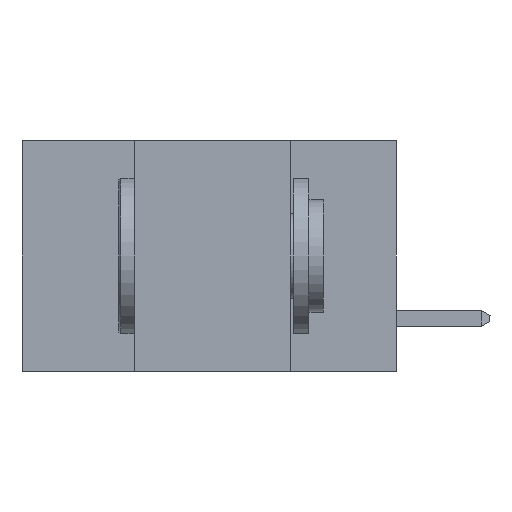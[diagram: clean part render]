
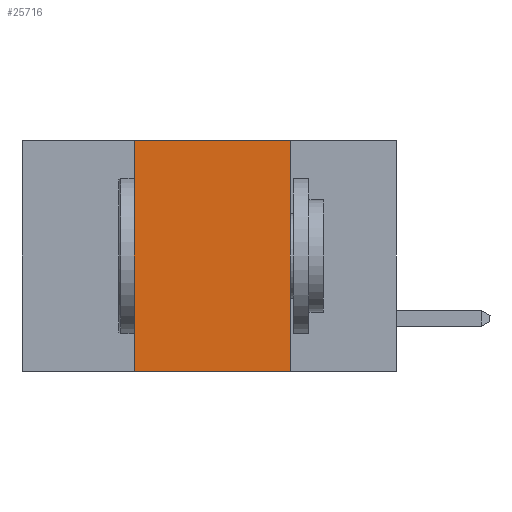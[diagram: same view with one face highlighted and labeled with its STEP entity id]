
A CAD part, left-side view. The second image highlights one B-rep face of the part: STEP entity #25716.
In plain terms, the highlighted planar face has unit normal (-1, 0, 0).
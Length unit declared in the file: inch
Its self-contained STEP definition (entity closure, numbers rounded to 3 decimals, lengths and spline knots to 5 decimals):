
#216 = DIRECTION ( 'NONE',  ( 1., 0., 0. ) ) ;
#978 = EDGE_LOOP ( 'NONE', ( #2393, #16390, #19862, #27914 ) ) ;
#1109 = EDGE_CURVE ( 'NONE', #26123, #24449, #20976, .T. ) ;
#1165 = LINE ( 'NONE', #5066, #31692 ) ;
#2374 = DIRECTION ( 'NONE',  ( 0., 0., -1. ) ) ;
#2393 = ORIENTED_EDGE ( 'NONE', *, *, #22762, .F. ) ;
#3804 = LINE ( 'NONE', #12162, #8048 ) ;
#5066 = CARTESIAN_POINT ( 'NONE',  ( 0., 0.6, 0. ) ) ;
#6222 = AXIS2_PLACEMENT_3D ( 'NONE', #26972, #216, #2374 ) ;
#8048 = VECTOR ( 'NONE', #26833, 39.37008 ) ;
#9158 = FACE_OUTER_BOUND ( 'NONE', #978, .T. ) ;
#9407 = CARTESIAN_POINT ( 'NONE',  ( 0., 0.6, -0.37 ) ) ;
#9566 = EDGE_CURVE ( 'NONE', #30830, #19050, #1165, .T. ) ;
#9730 = PLANE ( 'NONE',  #6222 ) ;
#10147 = VECTOR ( 'NONE', #14366, 39.37008 ) ;
#10358 = CARTESIAN_POINT ( 'NONE',  ( 0., 0.17, 0. ) ) ;
#12120 = DIRECTION ( 'NONE',  ( 0., 0., -1. ) ) ;
#12162 = CARTESIAN_POINT ( 'NONE',  ( 0., 0.42, 0. ) ) ;
#12281 = DIRECTION ( 'NONE',  ( 0., -1., 0. ) ) ;
#14366 = DIRECTION ( 'NONE',  ( 0., -1., 0. ) ) ;
#14798 = VECTOR ( 'NONE', #12120, 39.37008 ) ;
#15199 = CARTESIAN_POINT ( 'NONE',  ( 0., 0.17, -0.37 ) ) ;
#16390 = ORIENTED_EDGE ( 'NONE', *, *, #9566, .F. ) ;
#17974 = EDGE_CURVE ( 'NONE', #26123, #30830, #3804, .T. ) ;
#19050 = VERTEX_POINT ( 'NONE', #10358 ) ;
#19807 = CARTESIAN_POINT ( 'NONE',  ( 0., 0.42, 0. ) ) ;
#19862 = ORIENTED_EDGE ( 'NONE', *, *, #17974, .F. ) ;
#20976 = LINE ( 'NONE', #9407, #10147 ) ;
#22762 = EDGE_CURVE ( 'NONE', #19050, #24449, #27917, .T. ) ;
#24449 = VERTEX_POINT ( 'NONE', #15199 ) ;
#25716 = ADVANCED_FACE ( 'NONE', ( #9158 ), #9730, .F. ) ;
#26123 = VERTEX_POINT ( 'NONE', #31371 ) ;
#26833 = DIRECTION ( 'NONE',  ( 0., 0., 1. ) ) ;
#26972 = CARTESIAN_POINT ( 'NONE',  ( 0., 0.6, 0. ) ) ;
#27914 = ORIENTED_EDGE ( 'NONE', *, *, #1109, .T. ) ;
#27917 = LINE ( 'NONE', #31799, #14798 ) ;
#30830 = VERTEX_POINT ( 'NONE', #19807 ) ;
#31371 = CARTESIAN_POINT ( 'NONE',  ( 0., 0.42, -0.37 ) ) ;
#31692 = VECTOR ( 'NONE', #12281, 39.37008 ) ;
#31799 = CARTESIAN_POINT ( 'NONE',  ( 0., 0.17, 0. ) ) ;
